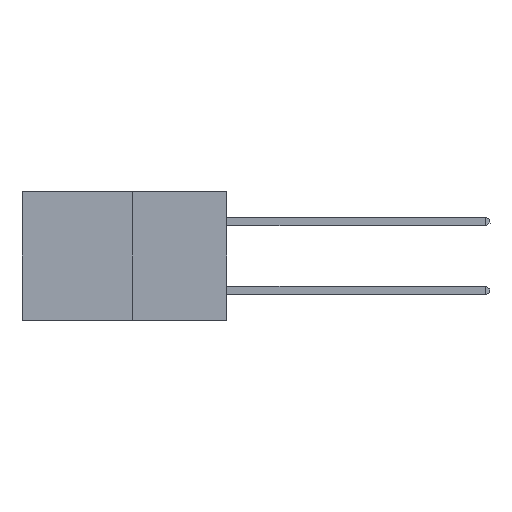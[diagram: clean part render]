
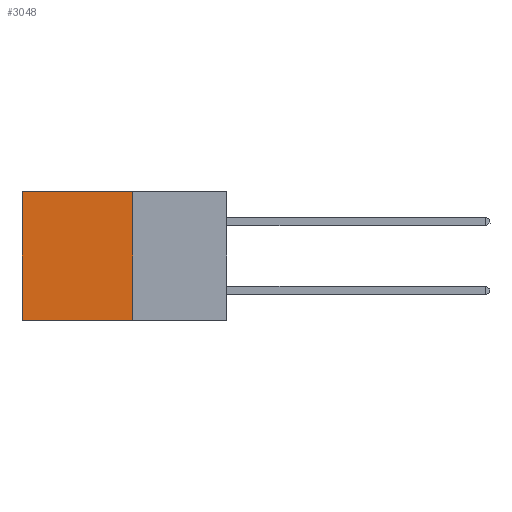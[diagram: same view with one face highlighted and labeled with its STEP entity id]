
A CAD part, left-side view. The second image highlights one B-rep face of the part: STEP entity #3048.
In plain terms, the highlighted planar face has unit normal (-1, 0, 0).
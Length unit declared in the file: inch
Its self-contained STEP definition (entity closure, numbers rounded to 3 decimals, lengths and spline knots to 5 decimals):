
#95 = EDGE_LOOP ( 'NONE', ( #1892, #7885, #1583, #3992 ) ) ;
#101 = EDGE_CURVE ( 'NONE', #7112, #7717, #7106, .T. ) ;
#214 = CARTESIAN_POINT ( 'NONE',  ( 0.277, 0.27, -0.37 ) ) ;
#294 = CARTESIAN_POINT ( 'NONE',  ( 0.277, 0.27, -0.37 ) ) ;
#364 = AXIS2_PLACEMENT_3D ( 'NONE', #294, #7929, #7947 ) ;
#672 = VERTEX_POINT ( 'NONE', #214 ) ;
#1227 = VECTOR ( 'NONE', #7324, 39.37008 ) ;
#1407 = VERTEX_POINT ( 'NONE', #6786 ) ;
#1583 = ORIENTED_EDGE ( 'NONE', *, *, #1740, .F. ) ;
#1723 = CARTESIAN_POINT ( 'NONE',  ( 0.277, 0.27, -0.37 ) ) ;
#1740 = EDGE_CURVE ( 'NONE', #7112, #672, #3139, .T. ) ;
#1750 = EDGE_CURVE ( 'NONE', #672, #1407, #6241, .T. ) ;
#1892 = ORIENTED_EDGE ( 'NONE', *, *, #5346, .T. ) ;
#2386 = DIRECTION ( 'NONE',  ( 0., 1., 0. ) ) ;
#2576 = CARTESIAN_POINT ( 'NONE',  ( 0.277, 0.27, 0. ) ) ;
#2782 = DIRECTION ( 'NONE',  ( 0., 0., -1. ) ) ;
#3048 = ADVANCED_FACE ( 'NONE', ( #7931 ), #7282, .F. ) ;
#3139 = LINE ( 'NONE', #1723, #1227 ) ;
#3925 = CARTESIAN_POINT ( 'NONE',  ( 0.277, 0.59, 0. ) ) ;
#3992 = ORIENTED_EDGE ( 'NONE', *, *, #101, .T. ) ;
#4117 = CARTESIAN_POINT ( 'NONE',  ( 0.277, 0.27, 0. ) ) ;
#4638 = VECTOR ( 'NONE', #6966, 39.37008 ) ;
#4738 = CARTESIAN_POINT ( 'NONE',  ( 0.277, 0.59, -0.37 ) ) ;
#5346 = EDGE_CURVE ( 'NONE', #7717, #1407, #7486, .T. ) ;
#5515 = VECTOR ( 'NONE', #2386, 39.37008 ) ;
#6241 = LINE ( 'NONE', #7466, #4638 ) ;
#6786 = CARTESIAN_POINT ( 'NONE',  ( 0.277, 0.59, -0.37 ) ) ;
#6966 = DIRECTION ( 'NONE',  ( 0., 1., 0. ) ) ;
#7106 = LINE ( 'NONE', #2576, #5515 ) ;
#7112 = VERTEX_POINT ( 'NONE', #4117 ) ;
#7282 = PLANE ( 'NONE',  #364 ) ;
#7305 = VECTOR ( 'NONE', #2782, 39.37008 ) ;
#7324 = DIRECTION ( 'NONE',  ( 0., 0., -1. ) ) ;
#7466 = CARTESIAN_POINT ( 'NONE',  ( 0.277, 0.27, -0.37 ) ) ;
#7486 = LINE ( 'NONE', #4738, #7305 ) ;
#7717 = VERTEX_POINT ( 'NONE', #3925 ) ;
#7885 = ORIENTED_EDGE ( 'NONE', *, *, #1750, .F. ) ;
#7929 = DIRECTION ( 'NONE',  ( 1., 0., 0. ) ) ;
#7931 = FACE_OUTER_BOUND ( 'NONE', #95, .T. ) ;
#7947 = DIRECTION ( 'NONE',  ( 0., 0., -1. ) ) ;
